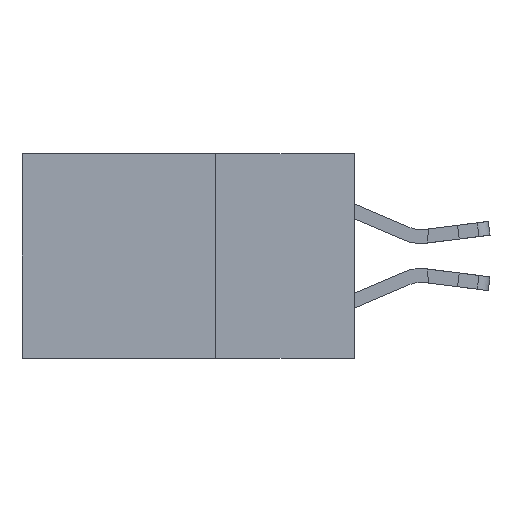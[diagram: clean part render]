
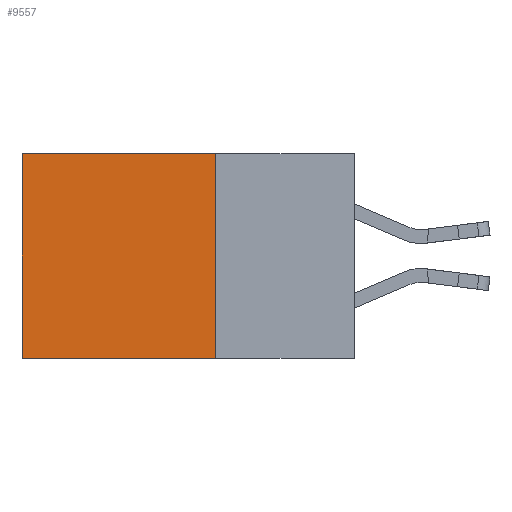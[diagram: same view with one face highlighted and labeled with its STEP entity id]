
A CAD part, left-side view. The second image highlights one B-rep face of the part: STEP entity #9557.
In plain terms, the highlighted planar face has unit normal (-1, 0, 0).
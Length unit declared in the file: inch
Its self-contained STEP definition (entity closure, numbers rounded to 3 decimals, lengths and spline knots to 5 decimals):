
#442 = ORIENTED_EDGE ( 'NONE', *, *, #19584, .T. ) ;
#1065 = DIRECTION ( 'NONE',  ( 0., 1., 0. ) ) ;
#3238 = EDGE_CURVE ( 'NONE', #12757, #20222, #9603, .T. ) ;
#5441 = DIRECTION ( 'NONE',  ( 0., 0., -1. ) ) ;
#5799 = CARTESIAN_POINT ( 'NONE',  ( 0.298, 0.25, -0.37 ) ) ;
#8059 = EDGE_LOOP ( 'NONE', ( #442, #24880, #23860, #19753 ) ) ;
#8991 = CARTESIAN_POINT ( 'NONE',  ( 0.298, 0.25, 0. ) ) ;
#9557 = ADVANCED_FACE ( 'NONE', ( #23294 ), #21530, .F. ) ;
#9603 = LINE ( 'NONE', #5799, #14262 ) ;
#10493 = CARTESIAN_POINT ( 'NONE',  ( 0.298, 0.25, 0. ) ) ;
#10919 = CARTESIAN_POINT ( 'NONE',  ( 0.298, 0.6, 0. ) ) ;
#10987 = DIRECTION ( 'NONE',  ( 0., 0., -1. ) ) ;
#11008 = VERTEX_POINT ( 'NONE', #14202 ) ;
#11775 = DIRECTION ( 'NONE',  ( 0., 1., 0. ) ) ;
#12757 = VERTEX_POINT ( 'NONE', #15182 ) ;
#13581 = DIRECTION ( 'NONE',  ( 0., 0., -1. ) ) ;
#13874 = VECTOR ( 'NONE', #1065, 39.37008 ) ;
#14202 = CARTESIAN_POINT ( 'NONE',  ( 0.298, 0.25, 0. ) ) ;
#14262 = VECTOR ( 'NONE', #11775, 39.37008 ) ;
#14864 = LINE ( 'NONE', #17363, #18930 ) ;
#15041 = CARTESIAN_POINT ( 'NONE',  ( 0.298, 0.6, -0.37 ) ) ;
#15182 = CARTESIAN_POINT ( 'NONE',  ( 0.298, 0.25, -0.37 ) ) ;
#17257 = AXIS2_PLACEMENT_3D ( 'NONE', #23564, #25597, #13581 ) ;
#17363 = CARTESIAN_POINT ( 'NONE',  ( 0.298, 0.6, 0. ) ) ;
#17570 = EDGE_CURVE ( 'NONE', #11008, #12757, #23925, .T. ) ;
#17950 = VECTOR ( 'NONE', #10987, 39.37008 ) ;
#18810 = VERTEX_POINT ( 'NONE', #10919 ) ;
#18930 = VECTOR ( 'NONE', #5441, 39.37008 ) ;
#19584 = EDGE_CURVE ( 'NONE', #18810, #20222, #14864, .T. ) ;
#19753 = ORIENTED_EDGE ( 'NONE', *, *, #20746, .T. ) ;
#20222 = VERTEX_POINT ( 'NONE', #15041 ) ;
#20746 = EDGE_CURVE ( 'NONE', #11008, #18810, #24538, .T. ) ;
#21530 = PLANE ( 'NONE',  #17257 ) ;
#23294 = FACE_OUTER_BOUND ( 'NONE', #8059, .T. ) ;
#23564 = CARTESIAN_POINT ( 'NONE',  ( 0.298, 0.25, 0. ) ) ;
#23860 = ORIENTED_EDGE ( 'NONE', *, *, #17570, .F. ) ;
#23925 = LINE ( 'NONE', #8991, #17950 ) ;
#24538 = LINE ( 'NONE', #10493, #13874 ) ;
#24880 = ORIENTED_EDGE ( 'NONE', *, *, #3238, .F. ) ;
#25597 = DIRECTION ( 'NONE',  ( 1., 0., 0. ) ) ;
